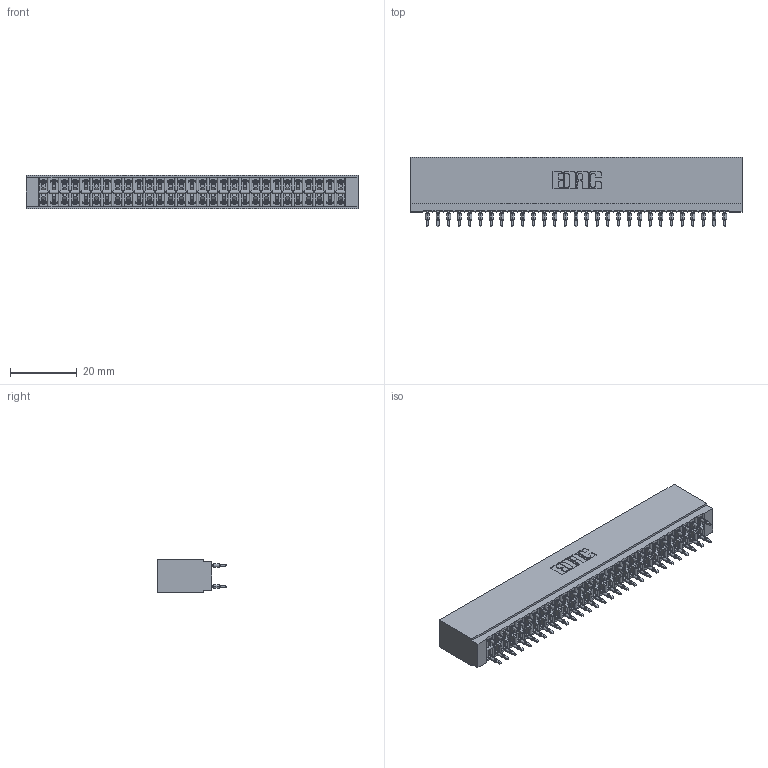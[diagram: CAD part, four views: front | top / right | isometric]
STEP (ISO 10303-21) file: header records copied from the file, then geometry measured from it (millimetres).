
FILE_DESCRIPTION (( 'STEP AP203' ), '1' );
FILE_NAME ('746-058-560-201.STEP', '2026-02-27T20:15:20', ( '' ), ( '' ), 'SwSTEP 2.0', 'SolidWorks 2023', '' );
FILE_SCHEMA (( 'CONFIG_CONTROL_DESIGN' ));
Length unit declared in the file: millimetre
Products named in the file (3): 746 Part_.515 Slot Depth - 01; 746-292-001_560; 746-058-560-201
Assembly tree (59 placements, depth 2):
  746-058-560-201
    746 Part_.515 Slot Depth - 01
    746-292-001_560  x58
Bounding box: 99.31 x 20.82 x 9.91 mm (x, y, z)
Volume: 10930 mm3; surface area: 18236 mm2
Topology: 59 solids, 59 shells, 5578 faces, 15517 edges, 9948 vertices
Faces by surface type: plane 2781, cylinder 1289, bspline 1160, torus 348
Entity records: 46774 total; most frequent: CARTESIAN_POINT 9409, ORIENTED_EDGE 8006, DIRECTION 6713, EDGE_CURVE 4003, LINE 3521, VECTOR 3521, VERTEX_POINT 2652, AXIS2_PLACEMENT_3D 1596
